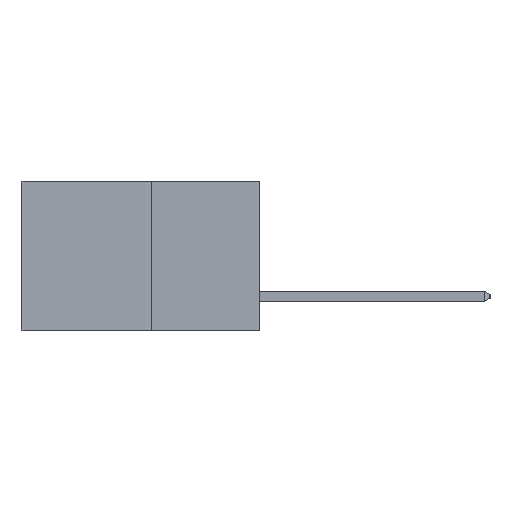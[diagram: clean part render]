
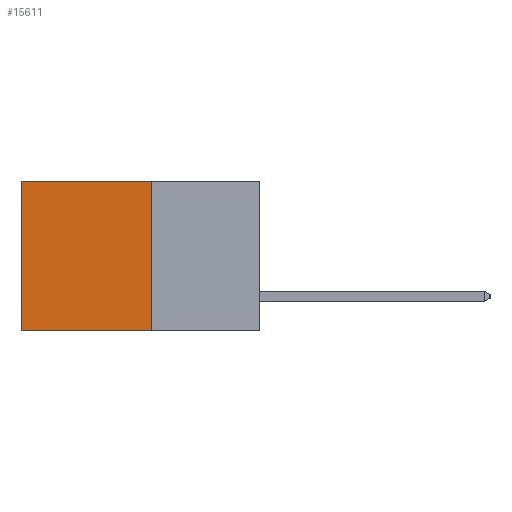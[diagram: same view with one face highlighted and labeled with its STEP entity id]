
A CAD part, left-side view. The second image highlights one B-rep face of the part: STEP entity #15611.
In plain terms, the highlighted planar face has unit normal (-1, 0, 0).
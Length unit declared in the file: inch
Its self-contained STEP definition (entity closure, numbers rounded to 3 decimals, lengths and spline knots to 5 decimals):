
#831 = CARTESIAN_POINT ( 'NONE',  ( 0.277, 0.27, -0.37 ) ) ;
#851 = CARTESIAN_POINT ( 'NONE',  ( 0.277, 0.59, -0.37 ) ) ;
#1098 = AXIS2_PLACEMENT_3D ( 'NONE', #24976, #2902, #18441 ) ;
#1165 = CARTESIAN_POINT ( 'NONE',  ( 0.277, 0.59, 0. ) ) ;
#2902 = DIRECTION ( 'NONE',  ( 1., 0., 0. ) ) ;
#3099 = DIRECTION ( 'NONE',  ( 0., 0., -1. ) ) ;
#4040 = VERTEX_POINT ( 'NONE', #1165 ) ;
#4304 = ORIENTED_EDGE ( 'NONE', *, *, #26739, .F. ) ;
#4422 = VECTOR ( 'NONE', #3099, 39.37008 ) ;
#5311 = EDGE_CURVE ( 'NONE', #20979, #4040, #19844, .T. ) ;
#5722 = FACE_OUTER_BOUND ( 'NONE', #18285, .T. ) ;
#5772 = DIRECTION ( 'NONE',  ( 0., 1., 0. ) ) ;
#6189 = VECTOR ( 'NONE', #13623, 39.37008 ) ;
#7738 = EDGE_CURVE ( 'NONE', #4040, #18858, #12810, .T. ) ;
#11419 = CARTESIAN_POINT ( 'NONE',  ( 0.277, 0.27, -0.37 ) ) ;
#11991 = ORIENTED_EDGE ( 'NONE', *, *, #7738, .T. ) ;
#12810 = LINE ( 'NONE', #20169, #6189 ) ;
#13306 = VECTOR ( 'NONE', #5772, 39.37008 ) ;
#13623 = DIRECTION ( 'NONE',  ( 0., 0., -1. ) ) ;
#14304 = VERTEX_POINT ( 'NONE', #11419 ) ;
#15611 = ADVANCED_FACE ( 'NONE', ( #5722 ), #16229, .F. ) ;
#16218 = LINE ( 'NONE', #18964, #26532 ) ;
#16229 = PLANE ( 'NONE',  #1098 ) ;
#17271 = ORIENTED_EDGE ( 'NONE', *, *, #5311, .T. ) ;
#18285 = EDGE_LOOP ( 'NONE', ( #11991, #4304, #25777, #17271 ) ) ;
#18441 = DIRECTION ( 'NONE',  ( 0., 0., -1. ) ) ;
#18858 = VERTEX_POINT ( 'NONE', #851 ) ;
#18964 = CARTESIAN_POINT ( 'NONE',  ( 0.277, 0.27, -0.37 ) ) ;
#19844 = LINE ( 'NONE', #25510, #13306 ) ;
#20169 = CARTESIAN_POINT ( 'NONE',  ( 0.277, 0.59, -0.37 ) ) ;
#20311 = EDGE_CURVE ( 'NONE', #20979, #14304, #22069, .T. ) ;
#20979 = VERTEX_POINT ( 'NONE', #21172 ) ;
#21144 = DIRECTION ( 'NONE',  ( 0., 1., 0. ) ) ;
#21172 = CARTESIAN_POINT ( 'NONE',  ( 0.277, 0.27, 0. ) ) ;
#22069 = LINE ( 'NONE', #831, #4422 ) ;
#24976 = CARTESIAN_POINT ( 'NONE',  ( 0.277, 0.27, -0.37 ) ) ;
#25510 = CARTESIAN_POINT ( 'NONE',  ( 0.277, 0.27, 0. ) ) ;
#25777 = ORIENTED_EDGE ( 'NONE', *, *, #20311, .F. ) ;
#26532 = VECTOR ( 'NONE', #21144, 39.37008 ) ;
#26739 = EDGE_CURVE ( 'NONE', #14304, #18858, #16218, .T. ) ;
